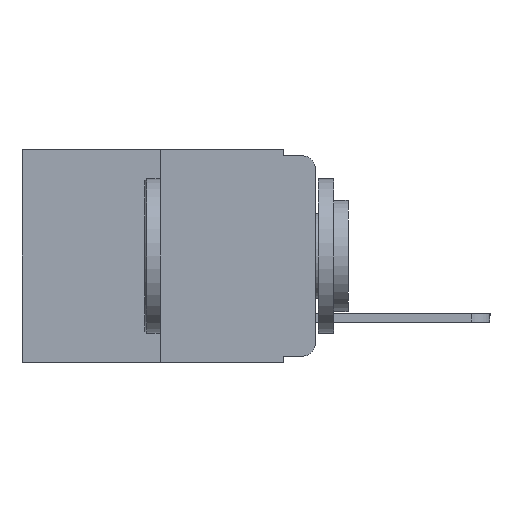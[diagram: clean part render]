
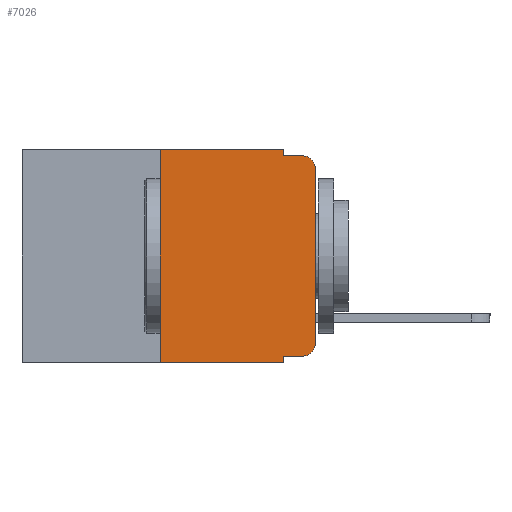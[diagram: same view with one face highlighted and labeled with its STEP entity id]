
A CAD part, left-side view. The second image highlights one B-rep face of the part: STEP entity #7026.
In plain terms, the highlighted planar face has unit normal (-1, 0, 0).
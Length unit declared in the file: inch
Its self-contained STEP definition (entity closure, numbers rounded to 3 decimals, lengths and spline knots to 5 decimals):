
#73 = DIRECTION ( 'NONE',  ( 0., 0., -1. ) ) ;
#150 = LINE ( 'NONE', #8988, #7694 ) ;
#414 = DIRECTION ( 'NONE',  ( 0., -1., 0. ) ) ;
#455 = VERTEX_POINT ( 'NONE', #11235 ) ;
#574 = CARTESIAN_POINT ( 'NONE',  ( 0., 0.02, -0.01 ) ) ;
#701 = VERTEX_POINT ( 'NONE', #3074 ) ;
#799 = LINE ( 'NONE', #7729, #8273 ) ;
#1027 = VERTEX_POINT ( 'NONE', #11297 ) ;
#1253 = VERTEX_POINT ( 'NONE', #2008 ) ;
#1449 = EDGE_LOOP ( 'NONE', ( #5852, #10765, #11047, #8964, #1874, #9524, #4724, #10732, #3512, #8620 ) ) ;
#1580 = EDGE_CURVE ( 'NONE', #1253, #1027, #3622, .T. ) ;
#1832 = EDGE_CURVE ( 'NONE', #4523, #4394, #799, .T. ) ;
#1874 = ORIENTED_EDGE ( 'NONE', *, *, #7471, .F. ) ;
#1971 = DIRECTION ( 'NONE',  ( 0., -1., 0. ) ) ;
#2008 = CARTESIAN_POINT ( 'NONE',  ( 0., 0.02, -0.333 ) ) ;
#2049 = DIRECTION ( 'NONE',  ( 0., 0., 1. ) ) ;
#2232 = EDGE_CURVE ( 'NONE', #3983, #8272, #4608, .T. ) ;
#2270 = FACE_OUTER_BOUND ( 'NONE', #1449, .T. ) ;
#3043 = DIRECTION ( 'NONE',  ( 0., 0., -1. ) ) ;
#3074 = CARTESIAN_POINT ( 'NONE',  ( 0., 0.25, 0. ) ) ;
#3092 = CARTESIAN_POINT ( 'NONE',  ( 0., 0.051, 0. ) ) ;
#3307 = DIRECTION ( 'NONE',  ( 0., -1., 0. ) ) ;
#3426 = CARTESIAN_POINT ( 'NONE',  ( 0., 0., 0. ) ) ;
#3512 = ORIENTED_EDGE ( 'NONE', *, *, #4398, .T. ) ;
#3622 = CIRCLE ( 'NONE', #9726, 0.02 ) ;
#3983 = VERTEX_POINT ( 'NONE', #10231 ) ;
#4021 = VECTOR ( 'NONE', #1971, 39.37008 ) ;
#4194 = CARTESIAN_POINT ( 'NONE',  ( 0., 0.051, -0.333 ) ) ;
#4394 = VERTEX_POINT ( 'NONE', #11701 ) ;
#4398 = EDGE_CURVE ( 'NONE', #4523, #1253, #7331, .T. ) ;
#4435 = CARTESIAN_POINT ( 'NONE',  ( 0., 0.051, -0.333 ) ) ;
#4523 = VERTEX_POINT ( 'NONE', #4435 ) ;
#4608 = LINE ( 'NONE', #9621, #4021 ) ;
#4698 = VECTOR ( 'NONE', #3307, 39.37008 ) ;
#4724 = ORIENTED_EDGE ( 'NONE', *, *, #9566, .T. ) ;
#5342 = CARTESIAN_POINT ( 'NONE',  ( 0., 0.02, -0.03 ) ) ;
#5344 = CARTESIAN_POINT ( 'NONE',  ( 0., 0.02, -0.313 ) ) ;
#5441 = VECTOR ( 'NONE', #2049, 39.37008 ) ;
#5502 = DIRECTION ( 'NONE',  ( 1., 0., 0. ) ) ;
#5852 = ORIENTED_EDGE ( 'NONE', *, *, #6344, .T. ) ;
#5985 = CIRCLE ( 'NONE', #9863, 0.02 ) ;
#6335 = DIRECTION ( 'NONE',  ( 0., 0., -1. ) ) ;
#6344 = EDGE_CURVE ( 'NONE', #1027, #6744, #9747, .T. ) ;
#6445 = PLANE ( 'NONE',  #7206 ) ;
#6744 = VERTEX_POINT ( 'NONE', #6944 ) ;
#6944 = CARTESIAN_POINT ( 'NONE',  ( 0., 0., -0.03 ) ) ;
#7026 = ADVANCED_FACE ( 'NONE', ( #2270 ), #6445, .F. ) ;
#7206 = AXIS2_PLACEMENT_3D ( 'NONE', #11051, #5502, #11975 ) ;
#7331 = LINE ( 'NONE', #4194, #4698 ) ;
#7471 = EDGE_CURVE ( 'NONE', #701, #8505, #150, .T. ) ;
#7694 = VECTOR ( 'NONE', #414, 39.37008 ) ;
#7729 = CARTESIAN_POINT ( 'NONE',  ( 0., 0.051, 0. ) ) ;
#7834 = CARTESIAN_POINT ( 'NONE',  ( 0., 0.25, 0. ) ) ;
#7995 = LINE ( 'NONE', #7834, #5441 ) ;
#8272 = VERTEX_POINT ( 'NONE', #574 ) ;
#8273 = VECTOR ( 'NONE', #8506, 39.37008 ) ;
#8437 = CARTESIAN_POINT ( 'NONE',  ( 0., 0.473, -0.343 ) ) ;
#8505 = VERTEX_POINT ( 'NONE', #12334 ) ;
#8506 = DIRECTION ( 'NONE',  ( 0., 0., -1. ) ) ;
#8620 = ORIENTED_EDGE ( 'NONE', *, *, #1580, .T. ) ;
#8812 = VECTOR ( 'NONE', #9381, 39.37008 ) ;
#8964 = ORIENTED_EDGE ( 'NONE', *, *, #10363, .F. ) ;
#8988 = CARTESIAN_POINT ( 'NONE',  ( 0., 0.473, 0. ) ) ;
#9381 = DIRECTION ( 'NONE',  ( 0., -1., 0. ) ) ;
#9390 = LINE ( 'NONE', #8437, #8812 ) ;
#9519 = VECTOR ( 'NONE', #73, 39.37008 ) ;
#9524 = ORIENTED_EDGE ( 'NONE', *, *, #11555, .F. ) ;
#9566 = EDGE_CURVE ( 'NONE', #455, #4394, #9390, .T. ) ;
#9621 = CARTESIAN_POINT ( 'NONE',  ( 0., 0.051, -0.01 ) ) ;
#9715 = DIRECTION ( 'NONE',  ( -1., 0., 0. ) ) ;
#9726 = AXIS2_PLACEMENT_3D ( 'NONE', #5344, #9715, #3043 ) ;
#9747 = LINE ( 'NONE', #3426, #11835 ) ;
#9863 = AXIS2_PLACEMENT_3D ( 'NONE', #5342, #11828, #6335 ) ;
#10053 = EDGE_CURVE ( 'NONE', #6744, #8272, #5985, .T. ) ;
#10073 = DIRECTION ( 'NONE',  ( 0., 0., 1. ) ) ;
#10231 = CARTESIAN_POINT ( 'NONE',  ( 0., 0.051, -0.01 ) ) ;
#10363 = EDGE_CURVE ( 'NONE', #8505, #3983, #11897, .T. ) ;
#10732 = ORIENTED_EDGE ( 'NONE', *, *, #1832, .F. ) ;
#10765 = ORIENTED_EDGE ( 'NONE', *, *, #10053, .T. ) ;
#11047 = ORIENTED_EDGE ( 'NONE', *, *, #2232, .F. ) ;
#11051 = CARTESIAN_POINT ( 'NONE',  ( 0., 0.473, 0. ) ) ;
#11235 = CARTESIAN_POINT ( 'NONE',  ( 0., 0.25, -0.343 ) ) ;
#11297 = CARTESIAN_POINT ( 'NONE',  ( 0., 0., -0.313 ) ) ;
#11555 = EDGE_CURVE ( 'NONE', #455, #701, #7995, .T. ) ;
#11701 = CARTESIAN_POINT ( 'NONE',  ( 0., 0.051, -0.343 ) ) ;
#11828 = DIRECTION ( 'NONE',  ( -1., 0., 0. ) ) ;
#11835 = VECTOR ( 'NONE', #10073, 39.37008 ) ;
#11897 = LINE ( 'NONE', #3092, #9519 ) ;
#11975 = DIRECTION ( 'NONE',  ( 0., 0., -1. ) ) ;
#12334 = CARTESIAN_POINT ( 'NONE',  ( 0., 0.051, 0. ) ) ;
